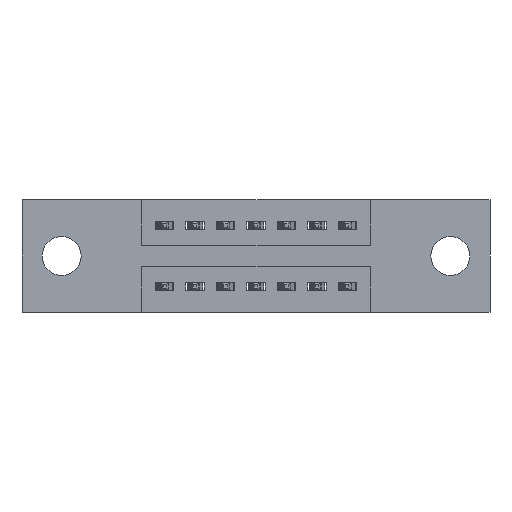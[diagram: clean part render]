
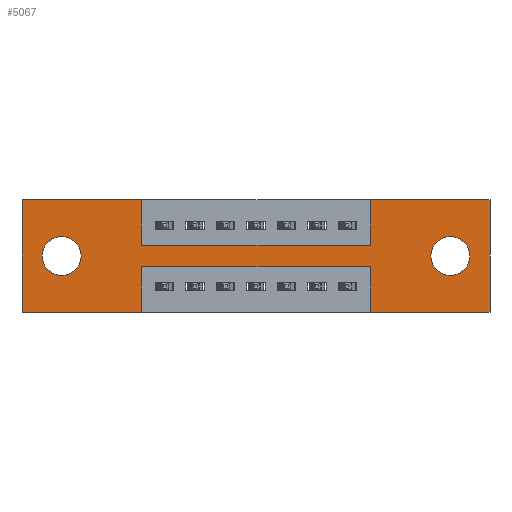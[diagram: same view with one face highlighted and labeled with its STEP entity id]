
A CAD part, front view. The second image highlights one B-rep face of the part: STEP entity #5067.
In plain terms, the highlighted planar face has unit normal (0, -1, 0).
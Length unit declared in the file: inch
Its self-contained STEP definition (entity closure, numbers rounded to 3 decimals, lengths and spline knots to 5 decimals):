
#2 = EDGE_CURVE ( 'NONE', #7172, #4923, #7605, .T. ) ;
#208 = ORIENTED_EDGE ( 'NONE', *, *, #2455, .F. ) ;
#244 = CARTESIAN_POINT ( 'NONE',  ( 0., 0., 0. ) ) ;
#286 = CARTESIAN_POINT ( 'NONE',  ( 0.3925, 0., 0. ) ) ;
#354 = DIRECTION ( 'NONE',  ( 0., 1., 0. ) ) ;
#377 = CARTESIAN_POINT ( 'NONE',  ( 1.1425, 0., -0.37 ) ) ;
#432 = EDGE_CURVE ( 'NONE', #6573, #3531, #6014, .T. ) ;
#490 = LINE ( 'NONE', #4333, #9241 ) ;
#595 = DIRECTION ( 'NONE',  ( -1., 0., 0. ) ) ;
#606 = CARTESIAN_POINT ( 'NONE',  ( 0.13, 0., -0.185 ) ) ;
#686 = CIRCLE ( 'NONE', #8182, 0.064 ) ;
#826 = CARTESIAN_POINT ( 'NONE',  ( 1.405, 0., -0.249 ) ) ;
#896 = ORIENTED_EDGE ( 'NONE', *, *, #2650, .F. ) ;
#1144 = DIRECTION ( 'NONE',  ( 0., 0., -1. ) ) ;
#1276 = DIRECTION ( 'NONE',  ( -1., 0., 0. ) ) ;
#1278 = CARTESIAN_POINT ( 'NONE',  ( 1.1425, 0., -0.22 ) ) ;
#1288 = CARTESIAN_POINT ( 'NONE',  ( 0.3925, 0., -0.15 ) ) ;
#1322 = EDGE_CURVE ( 'NONE', #8784, #2271, #686, .T. ) ;
#1384 = EDGE_CURVE ( 'NONE', #3747, #8692, #4758, .T. ) ;
#1448 = VECTOR ( 'NONE', #6001, 39.37008 ) ;
#1520 = CARTESIAN_POINT ( 'NONE',  ( 0.3925, 0., -0.22 ) ) ;
#1665 = VERTEX_POINT ( 'NONE', #244 ) ;
#1708 = FACE_BOUND ( 'NONE', #3654, .T. ) ;
#1841 = FACE_OUTER_BOUND ( 'NONE', #9120, .T. ) ;
#1856 = CARTESIAN_POINT ( 'NONE',  ( 0.3925, 0., -0.37 ) ) ;
#2141 = CARTESIAN_POINT ( 'NONE',  ( 0., 0., 0. ) ) ;
#2229 = CARTESIAN_POINT ( 'NONE',  ( 0., 0., -0.37 ) ) ;
#2271 = VERTEX_POINT ( 'NONE', #9243 ) ;
#2316 = LINE ( 'NONE', #2141, #4532 ) ;
#2321 = VERTEX_POINT ( 'NONE', #3078 ) ;
#2328 = CARTESIAN_POINT ( 'NONE',  ( 1.405, 0., -0.185 ) ) ;
#2438 = CARTESIAN_POINT ( 'NONE',  ( 1.535, 0., 0. ) ) ;
#2444 = EDGE_CURVE ( 'NONE', #2271, #8784, #8763, .T. ) ;
#2455 = EDGE_CURVE ( 'NONE', #4923, #3747, #490, .T. ) ;
#2548 = ORIENTED_EDGE ( 'NONE', *, *, #2444, .T. ) ;
#2564 = LINE ( 'NONE', #1288, #1448 ) ;
#2640 = EDGE_CURVE ( 'NONE', #7948, #6810, #3592, .T. ) ;
#2650 = EDGE_CURVE ( 'NONE', #7041, #6939, #5437, .T. ) ;
#2711 = EDGE_CURVE ( 'NONE', #6939, #7948, #7876, .T. ) ;
#2724 = VERTEX_POINT ( 'NONE', #377 ) ;
#2752 = ORIENTED_EDGE ( 'NONE', *, *, #2711, .F. ) ;
#2987 = PLANE ( 'NONE',  #9683 ) ;
#3078 = CARTESIAN_POINT ( 'NONE',  ( 0.3925, 0., -0.15 ) ) ;
#3277 = ORIENTED_EDGE ( 'NONE', *, *, #6541, .F. ) ;
#3353 = VECTOR ( 'NONE', #10206, 39.37008 ) ;
#3449 = DIRECTION ( 'NONE',  ( 0., 0., -1. ) ) ;
#3531 = VERTEX_POINT ( 'NONE', #826 ) ;
#3592 = LINE ( 'NONE', #2438, #6424 ) ;
#3599 = CARTESIAN_POINT ( 'NONE',  ( 0., 0., -0.37 ) ) ;
#3628 = CARTESIAN_POINT ( 'NONE',  ( 1.1425, 0., -0.37 ) ) ;
#3654 = EDGE_LOOP ( 'NONE', ( #5522, #2548 ) ) ;
#3747 = VERTEX_POINT ( 'NONE', #1856 ) ;
#3796 = EDGE_CURVE ( 'NONE', #2724, #7172, #6992, .T. ) ;
#3815 = VECTOR ( 'NONE', #6699, 39.37008 ) ;
#3916 = CARTESIAN_POINT ( 'NONE',  ( 1.535, 0., -0.37 ) ) ;
#3955 = EDGE_LOOP ( 'NONE', ( #4179, #8985 ) ) ;
#3981 = DIRECTION ( 'NONE',  ( 0., 1., 0. ) ) ;
#3999 = VECTOR ( 'NONE', #3449, 39.37008 ) ;
#4168 = LINE ( 'NONE', #9172, #8573 ) ;
#4179 = ORIENTED_EDGE ( 'NONE', *, *, #432, .T. ) ;
#4264 = DIRECTION ( 'NONE',  ( 0., 0., 1. ) ) ;
#4333 = CARTESIAN_POINT ( 'NONE',  ( 0.3925, 0., -0.37 ) ) ;
#4365 = LINE ( 'NONE', #286, #3999 ) ;
#4532 = VECTOR ( 'NONE', #9312, 39.37008 ) ;
#4593 = AXIS2_PLACEMENT_3D ( 'NONE', #9735, #354, #4264 ) ;
#4624 = DIRECTION ( 'NONE',  ( 0., 0., 1. ) ) ;
#4635 = EDGE_CURVE ( 'NONE', #3531, #6573, #9336, .T. ) ;
#4666 = ORIENTED_EDGE ( 'NONE', *, *, #2640, .F. ) ;
#4679 = VECTOR ( 'NONE', #595, 39.37008 ) ;
#4758 = LINE ( 'NONE', #6648, #5749 ) ;
#4799 = CARTESIAN_POINT ( 'NONE',  ( 0., 0., 0. ) ) ;
#4871 = ORIENTED_EDGE ( 'NONE', *, *, #5533, .F. ) ;
#4923 = VERTEX_POINT ( 'NONE', #5321 ) ;
#4996 = CARTESIAN_POINT ( 'NONE',  ( 0., 0., -0.37 ) ) ;
#5067 = ADVANCED_FACE ( 'NONE', ( #10083, #1708, #1841 ), #2987, .T. ) ;
#5240 = VECTOR ( 'NONE', #1276, 39.37008 ) ;
#5321 = CARTESIAN_POINT ( 'NONE',  ( 0.3925, 0., -0.22 ) ) ;
#5437 = LINE ( 'NONE', #7808, #3353 ) ;
#5522 = ORIENTED_EDGE ( 'NONE', *, *, #1322, .T. ) ;
#5528 = EDGE_CURVE ( 'NONE', #1665, #5683, #2316, .T. ) ;
#5533 = EDGE_CURVE ( 'NONE', #8692, #1665, #4168, .T. ) ;
#5683 = VERTEX_POINT ( 'NONE', #6155 ) ;
#5749 = VECTOR ( 'NONE', #8954, 39.37008 ) ;
#5788 = CARTESIAN_POINT ( 'NONE',  ( 1.1425, 0., 0. ) ) ;
#5930 = CARTESIAN_POINT ( 'NONE',  ( 1.405, 0., -0.121 ) ) ;
#5992 = ORIENTED_EDGE ( 'NONE', *, *, #3796, .F. ) ;
#6001 = DIRECTION ( 'NONE',  ( 1., 0., 0. ) ) ;
#6014 = CIRCLE ( 'NONE', #9651, 0.064 ) ;
#6155 = CARTESIAN_POINT ( 'NONE',  ( 0.3925, 0., 0. ) ) ;
#6203 = EDGE_CURVE ( 'NONE', #2321, #7041, #2564, .T. ) ;
#6403 = ORIENTED_EDGE ( 'NONE', *, *, #1384, .F. ) ;
#6424 = VECTOR ( 'NONE', #7843, 39.37008 ) ;
#6464 = CARTESIAN_POINT ( 'NONE',  ( 1.405, 0., -0.185 ) ) ;
#6541 = EDGE_CURVE ( 'NONE', #6810, #2724, #7315, .T. ) ;
#6573 = VERTEX_POINT ( 'NONE', #5930 ) ;
#6648 = CARTESIAN_POINT ( 'NONE',  ( 0., 0., -0.37 ) ) ;
#6699 = DIRECTION ( 'NONE',  ( 0., 0., 1. ) ) ;
#6804 = ORIENTED_EDGE ( 'NONE', *, *, #7617, .F. ) ;
#6810 = VERTEX_POINT ( 'NONE', #3916 ) ;
#6939 = VERTEX_POINT ( 'NONE', #5788 ) ;
#6992 = LINE ( 'NONE', #3628, #3815 ) ;
#6995 = CARTESIAN_POINT ( 'NONE',  ( 0.13, 0., -0.121 ) ) ;
#7041 = VERTEX_POINT ( 'NONE', #8878 ) ;
#7172 = VERTEX_POINT ( 'NONE', #1278 ) ;
#7232 = DIRECTION ( 'NONE',  ( 0., 1., 0. ) ) ;
#7252 = ORIENTED_EDGE ( 'NONE', *, *, #5528, .F. ) ;
#7280 = DIRECTION ( 'NONE',  ( 1., 0., 0. ) ) ;
#7315 = LINE ( 'NONE', #4996, #5240 ) ;
#7605 = LINE ( 'NONE', #1520, #4679 ) ;
#7617 = EDGE_CURVE ( 'NONE', #5683, #2321, #4365, .T. ) ;
#7808 = CARTESIAN_POINT ( 'NONE',  ( 1.1425, 0., 0. ) ) ;
#7843 = DIRECTION ( 'NONE',  ( 0., 0., -1. ) ) ;
#7876 = LINE ( 'NONE', #4799, #8127 ) ;
#7948 = VERTEX_POINT ( 'NONE', #9882 ) ;
#8127 = VECTOR ( 'NONE', #7280, 39.37008 ) ;
#8182 = AXIS2_PLACEMENT_3D ( 'NONE', #606, #10092, #9311 ) ;
#8367 = ORIENTED_EDGE ( 'NONE', *, *, #2, .F. ) ;
#8573 = VECTOR ( 'NONE', #4624, 39.37008 ) ;
#8692 = VERTEX_POINT ( 'NONE', #2229 ) ;
#8763 = CIRCLE ( 'NONE', #4593, 0.064 ) ;
#8784 = VERTEX_POINT ( 'NONE', #6995 ) ;
#8878 = CARTESIAN_POINT ( 'NONE',  ( 1.1425, 0., -0.15 ) ) ;
#8954 = DIRECTION ( 'NONE',  ( -1., 0., 0. ) ) ;
#8985 = ORIENTED_EDGE ( 'NONE', *, *, #4635, .T. ) ;
#9079 = DIRECTION ( 'NONE',  ( 0., -1., 0. ) ) ;
#9120 = EDGE_LOOP ( 'NONE', ( #208, #8367, #5992, #3277, #4666, #2752, #896, #10108, #6804, #7252, #4871, #6403 ) ) ;
#9172 = CARTESIAN_POINT ( 'NONE',  ( 0., 0., 0. ) ) ;
#9241 = VECTOR ( 'NONE', #1144, 39.37008 ) ;
#9243 = CARTESIAN_POINT ( 'NONE',  ( 0.13, 0., -0.249 ) ) ;
#9311 = DIRECTION ( 'NONE',  ( 0., 0., 1. ) ) ;
#9312 = DIRECTION ( 'NONE',  ( 1., 0., 0. ) ) ;
#9336 = CIRCLE ( 'NONE', #10074, 0.064 ) ;
#9651 = AXIS2_PLACEMENT_3D ( 'NONE', #6464, #7232, #10007 ) ;
#9683 = AXIS2_PLACEMENT_3D ( 'NONE', #3599, #9079, #9892 ) ;
#9735 = CARTESIAN_POINT ( 'NONE',  ( 0.13, 0., -0.185 ) ) ;
#9882 = CARTESIAN_POINT ( 'NONE',  ( 1.535, 0., 0. ) ) ;
#9892 = DIRECTION ( 'NONE',  ( 0., 0., -1. ) ) ;
#10007 = DIRECTION ( 'NONE',  ( 0., 0., -1. ) ) ;
#10074 = AXIS2_PLACEMENT_3D ( 'NONE', #2328, #3981, #10242 ) ;
#10083 = FACE_BOUND ( 'NONE', #3955, .T. ) ;
#10092 = DIRECTION ( 'NONE',  ( 0., 1., 0. ) ) ;
#10108 = ORIENTED_EDGE ( 'NONE', *, *, #6203, .F. ) ;
#10206 = DIRECTION ( 'NONE',  ( 0., 0., 1. ) ) ;
#10242 = DIRECTION ( 'NONE',  ( 0., 0., -1. ) ) ;
